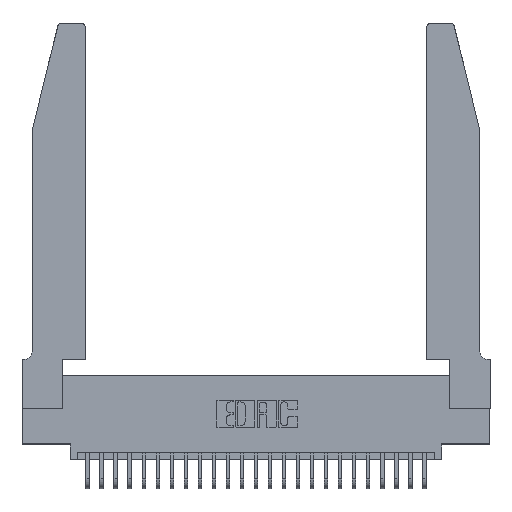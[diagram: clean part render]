
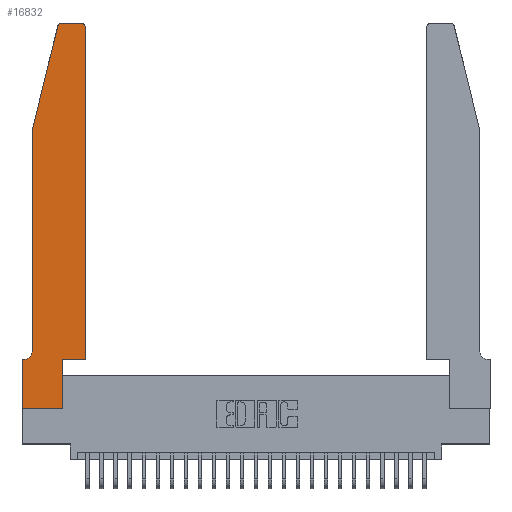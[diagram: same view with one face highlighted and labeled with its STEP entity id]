
A CAD part, top view. The second image highlights one B-rep face of the part: STEP entity #16832.
In plain terms, the highlighted planar face has unit normal (0, 0, 1).
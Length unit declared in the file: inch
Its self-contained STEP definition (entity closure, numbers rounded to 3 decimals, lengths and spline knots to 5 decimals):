
#724 = VERTEX_POINT ( 'NONE', #21061 ) ;
#1805 = VECTOR ( 'NONE', #14559, 39.37008 ) ;
#2175 = VECTOR ( 'NONE', #26801, 39.37008 ) ;
#2372 = VERTEX_POINT ( 'NONE', #5690 ) ;
#2430 = CIRCLE ( 'NONE', #8652, 0.07 ) ;
#3654 = CARTESIAN_POINT ( 'NONE',  ( 0.2865, 0., 0.37 ) ) ;
#3720 = DIRECTION ( 'NONE',  ( 0., 0., -1. ) ) ;
#3814 = CARTESIAN_POINT ( 'NONE',  ( 0.0055, 0.42, 0.37 ) ) ;
#3834 = LINE ( 'NONE', #6516, #13173 ) ;
#3911 = DIRECTION ( 'NONE',  ( -1., 0., 0. ) ) ;
#4013 = DIRECTION ( 'NONE',  ( 1., 0., 0. ) ) ;
#4502 = AXIS2_PLACEMENT_3D ( 'NONE', #8548, #12884, #14477 ) ;
#4815 = VERTEX_POINT ( 'NONE', #19450 ) ;
#4947 = EDGE_CURVE ( 'NONE', #27174, #5967, #7674, .T. ) ;
#4958 = EDGE_CURVE ( 'NONE', #12197, #9478, #18614, .T. ) ;
#5158 = EDGE_CURVE ( 'NONE', #9478, #4815, #3834, .T. ) ;
#5318 = VECTOR ( 'NONE', #18658, 39.37008 ) ;
#5567 = DIRECTION ( 'NONE',  ( 0., 0., 1. ) ) ;
#5690 = CARTESIAN_POINT ( 'NONE',  ( 0.25487, 2.72718, 0.37 ) ) ;
#5776 = EDGE_LOOP ( 'NONE', ( #26849, #8938, #27964, #14718, #20628, #18515, #26999, #8790, #23621, #8360, #17373, #22753 ) ) ;
#5967 = VERTEX_POINT ( 'NONE', #27036 ) ;
#6133 = DIRECTION ( 'NONE',  ( -1., 0., 0. ) ) ;
#6183 = DIRECTION ( 'NONE',  ( 0., -1., 0. ) ) ;
#6423 = DIRECTION ( 'NONE',  ( 1., 0., 0. ) ) ;
#6516 = CARTESIAN_POINT ( 'NONE',  ( 0.2865, 0.35, 0.37 ) ) ;
#7021 = CARTESIAN_POINT ( 'NONE',  ( 0., 0., 0.37 ) ) ;
#7674 = LINE ( 'NONE', #24417, #22794 ) ;
#8025 = CARTESIAN_POINT ( 'NONE',  ( 0.4205, 2.75, 0.37 ) ) ;
#8360 = ORIENTED_EDGE ( 'NONE', *, *, #21415, .T. ) ;
#8548 = CARTESIAN_POINT ( 'NONE',  ( 0.4205, 2.72, 0.37 ) ) ;
#8652 = AXIS2_PLACEMENT_3D ( 'NONE', #3814, #3720, #3911 ) ;
#8790 = ORIENTED_EDGE ( 'NONE', *, *, #4958, .T. ) ;
#8938 = ORIENTED_EDGE ( 'NONE', *, *, #9010, .T. ) ;
#9010 = EDGE_CURVE ( 'NONE', #14081, #2372, #24299, .T. ) ;
#9118 = CARTESIAN_POINT ( 'NONE',  ( 0.0755, 0.35, 0.37 ) ) ;
#9472 = CARTESIAN_POINT ( 'NONE',  ( 0., 0.35, 0.37 ) ) ;
#9478 = VERTEX_POINT ( 'NONE', #3654 ) ;
#9936 = AXIS2_PLACEMENT_3D ( 'NONE', #25253, #5567, #23508 ) ;
#10316 = VECTOR ( 'NONE', #24466, 39.37008 ) ;
#10757 = CARTESIAN_POINT ( 'NONE',  ( 0., 0.35, 0.37 ) ) ;
#11220 = EDGE_CURVE ( 'NONE', #20778, #14081, #21162, .T. ) ;
#12139 = EDGE_CURVE ( 'NONE', #2372, #27174, #28293, .T. ) ;
#12197 = VERTEX_POINT ( 'NONE', #7021 ) ;
#12234 = VECTOR ( 'NONE', #6133, 39.37008 ) ;
#12678 = PLANE ( 'NONE',  #28085 ) ;
#12795 = CARTESIAN_POINT ( 'NONE',  ( 0.4505, 0.35, 0.37 ) ) ;
#12884 = DIRECTION ( 'NONE',  ( 0., 0., 1. ) ) ;
#13173 = VECTOR ( 'NONE', #15323, 39.37008 ) ;
#14081 = VERTEX_POINT ( 'NONE', #18747 ) ;
#14477 = DIRECTION ( 'NONE',  ( 1., 0., 0. ) ) ;
#14559 = DIRECTION ( 'NONE',  ( -0.239, -0.971, 0. ) ) ;
#14562 = CARTESIAN_POINT ( 'NONE',  ( 0.4505, 0.35, 0.37 ) ) ;
#14718 = ORIENTED_EDGE ( 'NONE', *, *, #4947, .T. ) ;
#15095 = CARTESIAN_POINT ( 'NONE',  ( 0., 0., 0.37 ) ) ;
#15115 = EDGE_CURVE ( 'NONE', #724, #20778, #23624, .T. ) ;
#15323 = DIRECTION ( 'NONE',  ( 0., 1., 0. ) ) ;
#15465 = VERTEX_POINT ( 'NONE', #16086 ) ;
#15749 = CARTESIAN_POINT ( 'NONE',  ( 0., 0., 0.37 ) ) ;
#15851 = DIRECTION ( 'NONE',  ( 0., -1., 0. ) ) ;
#16086 = CARTESIAN_POINT ( 'NONE',  ( 0.0055, 0.35, 0.37 ) ) ;
#16832 = ADVANCED_FACE ( 'NONE', ( #22173 ), #12678, .T. ) ;
#17353 = DIRECTION ( 'NONE',  ( 0., 0., 1. ) ) ;
#17373 = ORIENTED_EDGE ( 'NONE', *, *, #25186, .T. ) ;
#18024 = VERTEX_POINT ( 'NONE', #18554 ) ;
#18515 = ORIENTED_EDGE ( 'NONE', *, *, #19786, .T. ) ;
#18554 = CARTESIAN_POINT ( 'NONE',  ( 0.4505, 0.35, 0.37 ) ) ;
#18614 = LINE ( 'NONE', #15749, #2175 ) ;
#18658 = DIRECTION ( 'NONE',  ( 0., 1., 0. ) ) ;
#18747 = CARTESIAN_POINT ( 'NONE',  ( 0.284, 2.75, 0.37 ) ) ;
#19450 = CARTESIAN_POINT ( 'NONE',  ( 0.2865, 0.35, 0.37 ) ) ;
#19786 = EDGE_CURVE ( 'NONE', #15465, #25493, #26797, .T. ) ;
#20628 = ORIENTED_EDGE ( 'NONE', *, *, #21354, .T. ) ;
#20778 = VERTEX_POINT ( 'NONE', #8025 ) ;
#20794 = CARTESIAN_POINT ( 'NONE',  ( 0.0755, 2., 0.37 ) ) ;
#21061 = CARTESIAN_POINT ( 'NONE',  ( 0.4505, 2.72, 0.37 ) ) ;
#21162 = LINE ( 'NONE', #21212, #12234 ) ;
#21212 = CARTESIAN_POINT ( 'NONE',  ( 0.2605, 2.75, 0.37 ) ) ;
#21260 = VECTOR ( 'NONE', #6183, 39.37008 ) ;
#21354 = EDGE_CURVE ( 'NONE', #5967, #15465, #2430, .T. ) ;
#21415 = EDGE_CURVE ( 'NONE', #4815, #18024, #24795, .T. ) ;
#21959 = LINE ( 'NONE', #15095, #21260 ) ;
#22173 = FACE_OUTER_BOUND ( 'NONE', #5776, .T. ) ;
#22717 = EDGE_CURVE ( 'NONE', #25493, #12197, #21959, .T. ) ;
#22753 = ORIENTED_EDGE ( 'NONE', *, *, #15115, .T. ) ;
#22794 = VECTOR ( 'NONE', #15851, 39.37008 ) ;
#23386 = CARTESIAN_POINT ( 'NONE',  ( 0.0755, 2., 0.37 ) ) ;
#23409 = VECTOR ( 'NONE', #4013, 39.37008 ) ;
#23508 = DIRECTION ( 'NONE',  ( 1., 0., 0. ) ) ;
#23621 = ORIENTED_EDGE ( 'NONE', *, *, #5158, .T. ) ;
#23624 = CIRCLE ( 'NONE', #4502, 0.03 ) ;
#24299 = CIRCLE ( 'NONE', #9936, 0.03 ) ;
#24417 = CARTESIAN_POINT ( 'NONE',  ( 0.0755, 2., 0.37 ) ) ;
#24466 = DIRECTION ( 'NONE',  ( -1., 0., 0. ) ) ;
#24795 = LINE ( 'NONE', #12795, #23409 ) ;
#25186 = EDGE_CURVE ( 'NONE', #18024, #724, #27696, .T. ) ;
#25253 = CARTESIAN_POINT ( 'NONE',  ( 0.284, 2.72, 0.37 ) ) ;
#25493 = VERTEX_POINT ( 'NONE', #9472 ) ;
#26797 = LINE ( 'NONE', #9118, #10316 ) ;
#26801 = DIRECTION ( 'NONE',  ( 1., 0., 0. ) ) ;
#26849 = ORIENTED_EDGE ( 'NONE', *, *, #11220, .T. ) ;
#26999 = ORIENTED_EDGE ( 'NONE', *, *, #22717, .T. ) ;
#27036 = CARTESIAN_POINT ( 'NONE',  ( 0.0755, 0.42, 0.37 ) ) ;
#27174 = VERTEX_POINT ( 'NONE', #23386 ) ;
#27696 = LINE ( 'NONE', #14562, #5318 ) ;
#27964 = ORIENTED_EDGE ( 'NONE', *, *, #12139, .T. ) ;
#28085 = AXIS2_PLACEMENT_3D ( 'NONE', #10757, #17353, #6423 ) ;
#28293 = LINE ( 'NONE', #20794, #1805 ) ;
